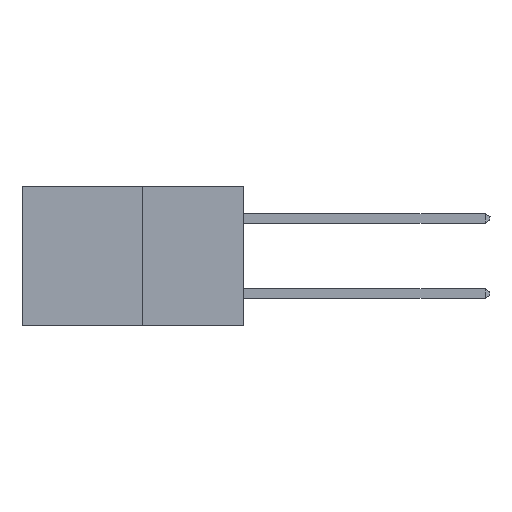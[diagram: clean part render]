
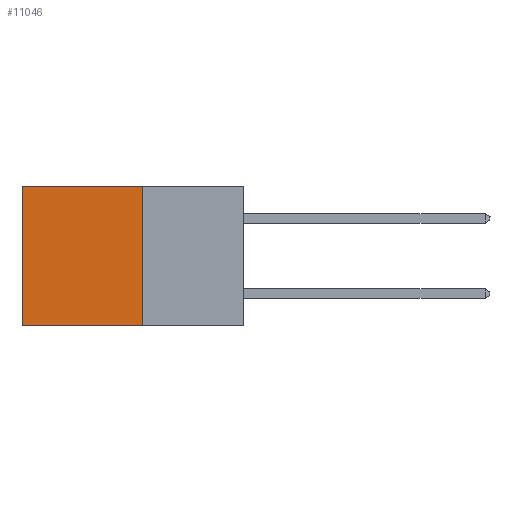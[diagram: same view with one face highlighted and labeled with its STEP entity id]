
A CAD part, left-side view. The second image highlights one B-rep face of the part: STEP entity #11046.
In plain terms, the highlighted planar face has unit normal (-1, 0, 0).
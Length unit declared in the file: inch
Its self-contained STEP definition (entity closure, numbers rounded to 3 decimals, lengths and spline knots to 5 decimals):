
#93 = CARTESIAN_POINT ( 'NONE',  ( 0.277, 0.27, -0.37 ) ) ;
#1016 = CARTESIAN_POINT ( 'NONE',  ( 0.277, 0.59, 0. ) ) ;
#1370 = EDGE_CURVE ( 'NONE', #8666, #6585, #8025, .T. ) ;
#1641 = ORIENTED_EDGE ( 'NONE', *, *, #6753, .T. ) ;
#2474 = ORIENTED_EDGE ( 'NONE', *, *, #8319, .F. ) ;
#2717 = CARTESIAN_POINT ( 'NONE',  ( 0.277, 0.27, 0. ) ) ;
#3342 = LINE ( 'NONE', #93, #8636 ) ;
#3699 = ORIENTED_EDGE ( 'NONE', *, *, #1370, .F. ) ;
#3709 = LINE ( 'NONE', #2717, #9010 ) ;
#4190 = DIRECTION ( 'NONE',  ( 0., 1., 0. ) ) ;
#4542 = VECTOR ( 'NONE', #5279, 39.37008 ) ;
#4556 = ORIENTED_EDGE ( 'NONE', *, *, #7459, .T. ) ;
#4838 = AXIS2_PLACEMENT_3D ( 'NONE', #5201, #5186, #5156 ) ;
#4913 = FACE_OUTER_BOUND ( 'NONE', #10773, .T. ) ;
#5156 = DIRECTION ( 'NONE',  ( 0., 0., -1. ) ) ;
#5186 = DIRECTION ( 'NONE',  ( 1., 0., 0. ) ) ;
#5201 = CARTESIAN_POINT ( 'NONE',  ( 0.277, 0.27, -0.37 ) ) ;
#5214 = PLANE ( 'NONE',  #4838 ) ;
#5279 = DIRECTION ( 'NONE',  ( 0., 0., -1. ) ) ;
#5287 = DIRECTION ( 'NONE',  ( 0., 1., 0. ) ) ;
#5716 = CARTESIAN_POINT ( 'NONE',  ( 0.277, 0.59, -0.37 ) ) ;
#5821 = CARTESIAN_POINT ( 'NONE',  ( 0.277, 0.59, -0.37 ) ) ;
#6585 = VERTEX_POINT ( 'NONE', #9759 ) ;
#6753 = EDGE_CURVE ( 'NONE', #11719, #7421, #12844, .T. ) ;
#7421 = VERTEX_POINT ( 'NONE', #5716 ) ;
#7459 = EDGE_CURVE ( 'NONE', #8666, #11719, #3709, .T. ) ;
#8025 = LINE ( 'NONE', #13139, #12572 ) ;
#8319 = EDGE_CURVE ( 'NONE', #6585, #7421, #3342, .T. ) ;
#8636 = VECTOR ( 'NONE', #5287, 39.37008 ) ;
#8666 = VERTEX_POINT ( 'NONE', #11926 ) ;
#9010 = VECTOR ( 'NONE', #4190, 39.37008 ) ;
#9759 = CARTESIAN_POINT ( 'NONE',  ( 0.277, 0.27, -0.37 ) ) ;
#9782 = DIRECTION ( 'NONE',  ( 0., 0., -1. ) ) ;
#10773 = EDGE_LOOP ( 'NONE', ( #1641, #2474, #3699, #4556 ) ) ;
#11046 = ADVANCED_FACE ( 'NONE', ( #4913 ), #5214, .F. ) ;
#11719 = VERTEX_POINT ( 'NONE', #1016 ) ;
#11926 = CARTESIAN_POINT ( 'NONE',  ( 0.277, 0.27, 0. ) ) ;
#12572 = VECTOR ( 'NONE', #9782, 39.37008 ) ;
#12844 = LINE ( 'NONE', #5821, #4542 ) ;
#13139 = CARTESIAN_POINT ( 'NONE',  ( 0.277, 0.27, -0.37 ) ) ;
